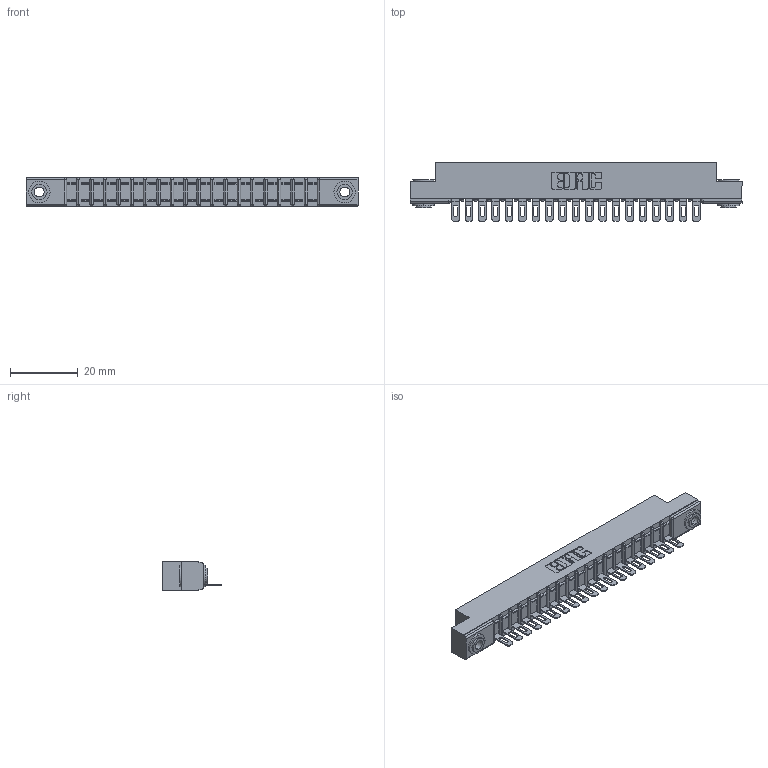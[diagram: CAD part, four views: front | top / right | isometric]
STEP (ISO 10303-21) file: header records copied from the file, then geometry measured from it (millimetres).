
FILE_DESCRIPTION (( 'STEP AP203' ), '1' );
FILE_NAME ('357-019-401-103.STEP', '2020-10-01T02:11:37', ( '' ), ( '' ), 'SwSTEP 2.0', 'SolidWorks 2020', '' );
FILE_SCHEMA (( 'CONFIG_CONTROL_DESIGN' ));
Length unit declared in the file: inch
Products named in the file (4): 345-250-002_345-250-002-102; 357-019-401-103; 307 Part_.156 Dia Mounting Holes; 307-290-002_501
Assembly tree (22 placements, depth 2):
  357-019-401-103
    307 Part_.156 Dia Mounting Holes
    307-290-002_501  x19
    345-250-002_345-250-002-102  x2
Bounding box: 98.3 x 17.42 x 8.71 mm (x, y, z)
Volume: 6505.7 mm3; surface area: 12037.8 mm2
Topology: 22 solids, 22 shells, 1634 faces, 4957 edges, 3246 vertices
Faces by surface type: plane 930, cylinder 656, sphere 40, cone 8
Entity records: 20983 total; most frequent: CARTESIAN_POINT 3513, ORIENTED_EDGE 3494, DIRECTION 3443, EDGE_CURVE 1747, LINE 1315, VECTOR 1315, VERTEX_POINT 1134, AXIS2_PLACEMENT_3D 1064
